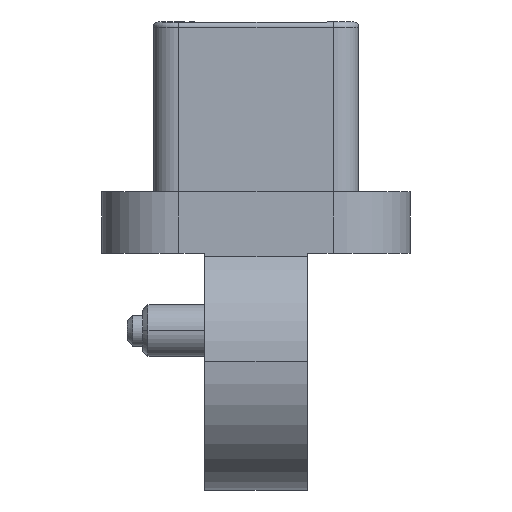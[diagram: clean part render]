
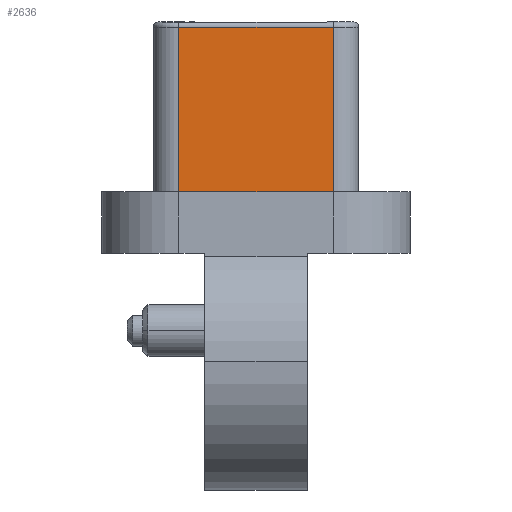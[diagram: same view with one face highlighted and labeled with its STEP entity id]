
A CAD part, left-side view. The second image highlights one B-rep face of the part: STEP entity #2636.
In plain terms, the highlighted planar face has unit normal (-1, 0, 0).
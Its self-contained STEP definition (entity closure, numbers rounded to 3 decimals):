
#247 = CARTESIAN_POINT ( 'NONE',  ( -8.45, 1.5, -0.1 ) ) ;
#392 = LINE ( 'NONE', #2839, #3574 ) ;
#702 = EDGE_CURVE ( 'NONE', #7214, #7011, #4419, .T. ) ;
#766 = VERTEX_POINT ( 'NONE', #5725 ) ;
#946 = CARTESIAN_POINT ( 'NONE',  ( -8.45, 0., -1.7 ) ) ;
#1375 = DIRECTION ( 'NONE',  ( 0., 0., 1. ) ) ;
#1703 = ORIENTED_EDGE ( 'NONE', *, *, #3001, .T. ) ;
#1996 = VECTOR ( 'NONE', #1375, 1000. ) ;
#2196 = EDGE_CURVE ( 'NONE', #7011, #3761, #2843, .T. ) ;
#2557 = ORIENTED_EDGE ( 'NONE', *, *, #5532, .T. ) ;
#2636 = ADVANCED_FACE ( 'NONE', ( #4004 ), #6534, .F. ) ;
#2686 = DIRECTION ( 'NONE',  ( 0., 0., -1. ) ) ;
#2698 = VECTOR ( 'NONE', #2686, 1000. ) ;
#2839 = CARTESIAN_POINT ( 'NONE',  ( -8.45, 1.5, -3.3 ) ) ;
#2843 = LINE ( 'NONE', #5317, #4309 ) ;
#3001 = EDGE_CURVE ( 'NONE', #3761, #766, #6431, .T. ) ;
#3401 = DIRECTION ( 'NONE',  ( 1., 0., 0. ) ) ;
#3574 = VECTOR ( 'NONE', #5313, 1000. ) ;
#3761 = VERTEX_POINT ( 'NONE', #4768 ) ;
#3896 = CARTESIAN_POINT ( 'NONE',  ( -8.45, -1.5, -0.1 ) ) ;
#4004 = FACE_OUTER_BOUND ( 'NONE', #5106, .T. ) ;
#4309 = VECTOR ( 'NONE', #7897, 1000. ) ;
#4419 = LINE ( 'NONE', #6982, #1996 ) ;
#4456 = ORIENTED_EDGE ( 'NONE', *, *, #2196, .T. ) ;
#4612 = ORIENTED_EDGE ( 'NONE', *, *, #702, .T. ) ;
#4661 = AXIS2_PLACEMENT_3D ( 'NONE', #946, #3401, #5880 ) ;
#4768 = CARTESIAN_POINT ( 'NONE',  ( -8.45, 1.5, -0.1 ) ) ;
#5106 = EDGE_LOOP ( 'NONE', ( #1703, #2557, #4612, #4456 ) ) ;
#5313 = DIRECTION ( 'NONE',  ( 0., -1., 0. ) ) ;
#5317 = CARTESIAN_POINT ( 'NONE',  ( -8.45, -1.5, -0.1 ) ) ;
#5532 = EDGE_CURVE ( 'NONE', #766, #7214, #392, .T. ) ;
#5725 = CARTESIAN_POINT ( 'NONE',  ( -8.45, 1.5, -3.3 ) ) ;
#5880 = DIRECTION ( 'NONE',  ( 0., 1., 0. ) ) ;
#6431 = LINE ( 'NONE', #247, #2698 ) ;
#6534 = PLANE ( 'NONE',  #4661 ) ;
#6855 = CARTESIAN_POINT ( 'NONE',  ( -8.45, -1.5, -3.3 ) ) ;
#6982 = CARTESIAN_POINT ( 'NONE',  ( -8.45, -1.5, -3.3 ) ) ;
#7011 = VERTEX_POINT ( 'NONE', #3896 ) ;
#7214 = VERTEX_POINT ( 'NONE', #6855 ) ;
#7897 = DIRECTION ( 'NONE',  ( 0., 1., 0. ) ) ;
